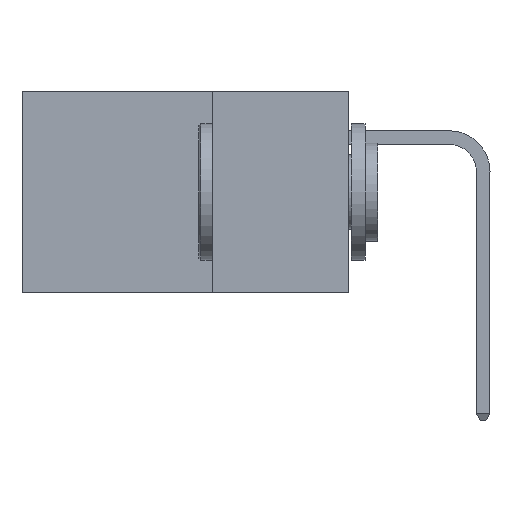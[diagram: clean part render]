
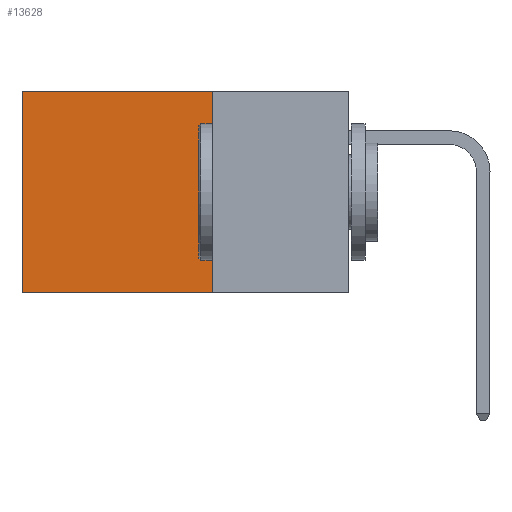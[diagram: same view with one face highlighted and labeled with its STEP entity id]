
A CAD part, left-side view. The second image highlights one B-rep face of the part: STEP entity #13628.
In plain terms, the highlighted planar face has unit normal (-1, 0, 0).
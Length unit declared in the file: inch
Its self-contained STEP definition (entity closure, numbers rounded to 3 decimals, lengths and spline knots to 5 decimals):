
#108 = VECTOR ( 'NONE', #14516, 39.37008 ) ;
#541 = CARTESIAN_POINT ( 'NONE',  ( 0.2875, 0.6, 0. ) ) ;
#639 = LINE ( 'NONE', #7973, #11650 ) ;
#1850 = ORIENTED_EDGE ( 'NONE', *, *, #12373, .F. ) ;
#1989 = VECTOR ( 'NONE', #7336, 39.37008 ) ;
#2013 = CARTESIAN_POINT ( 'NONE',  ( 0.2875, 0.25, 0. ) ) ;
#2288 = EDGE_CURVE ( 'NONE', #7378, #2691, #639, .T. ) ;
#2338 = EDGE_CURVE ( 'NONE', #2377, #11778, #5102, .T. ) ;
#2377 = VERTEX_POINT ( 'NONE', #7048 ) ;
#2691 = VERTEX_POINT ( 'NONE', #3614 ) ;
#3223 = AXIS2_PLACEMENT_3D ( 'NONE', #2013, #11327, #4374 ) ;
#3614 = CARTESIAN_POINT ( 'NONE',  ( 0.2875, 0.6, -0.37 ) ) ;
#4374 = DIRECTION ( 'NONE',  ( 0., 0., -1. ) ) ;
#5102 = LINE ( 'NONE', #7405, #1989 ) ;
#6455 = LINE ( 'NONE', #13421, #108 ) ;
#6544 = FACE_OUTER_BOUND ( 'NONE', #14950, .T. ) ;
#6592 = VECTOR ( 'NONE', #12466, 39.37008 ) ;
#7048 = CARTESIAN_POINT ( 'NONE',  ( 0.2875, 0.25, 0. ) ) ;
#7336 = DIRECTION ( 'NONE',  ( 0., 0., -1. ) ) ;
#7378 = VERTEX_POINT ( 'NONE', #541 ) ;
#7405 = CARTESIAN_POINT ( 'NONE',  ( 0.2875, 0.25, 0. ) ) ;
#7885 = DIRECTION ( 'NONE',  ( 0., 0., -1. ) ) ;
#7953 = CARTESIAN_POINT ( 'NONE',  ( 0.2875, 0.25, -0.37 ) ) ;
#7973 = CARTESIAN_POINT ( 'NONE',  ( 0.2875, 0.6, 0. ) ) ;
#8729 = ORIENTED_EDGE ( 'NONE', *, *, #2288, .T. ) ;
#10187 = PLANE ( 'NONE',  #3223 ) ;
#11314 = CARTESIAN_POINT ( 'NONE',  ( 0.2875, 0.25, -0.37 ) ) ;
#11327 = DIRECTION ( 'NONE',  ( 1., 0., 0. ) ) ;
#11509 = EDGE_CURVE ( 'NONE', #2377, #7378, #6455, .T. ) ;
#11650 = VECTOR ( 'NONE', #7885, 39.37008 ) ;
#11778 = VERTEX_POINT ( 'NONE', #7953 ) ;
#11874 = ORIENTED_EDGE ( 'NONE', *, *, #2338, .F. ) ;
#12373 = EDGE_CURVE ( 'NONE', #11778, #2691, #12723, .T. ) ;
#12466 = DIRECTION ( 'NONE',  ( 0., 1., 0. ) ) ;
#12723 = LINE ( 'NONE', #11314, #6592 ) ;
#13421 = CARTESIAN_POINT ( 'NONE',  ( 0.2875, 0.25, 0. ) ) ;
#13431 = ORIENTED_EDGE ( 'NONE', *, *, #11509, .T. ) ;
#13628 = ADVANCED_FACE ( 'NONE', ( #6544 ), #10187, .F. ) ;
#14516 = DIRECTION ( 'NONE',  ( 0., 1., 0. ) ) ;
#14950 = EDGE_LOOP ( 'NONE', ( #8729, #1850, #11874, #13431 ) ) ;
